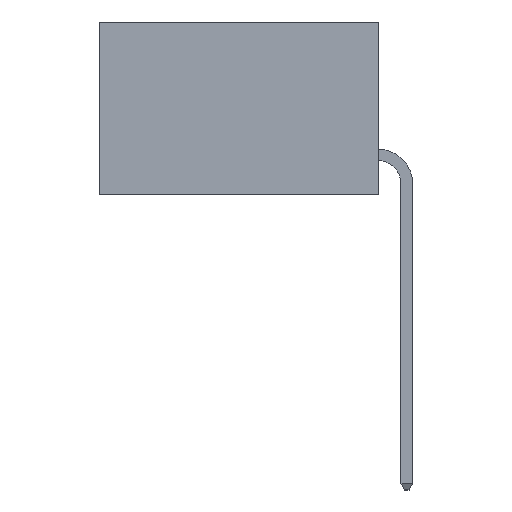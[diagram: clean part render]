
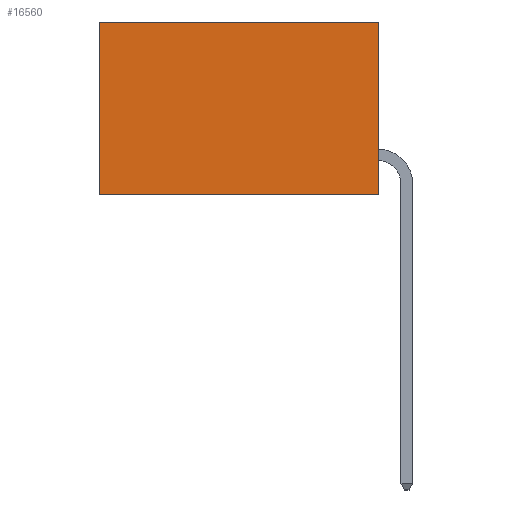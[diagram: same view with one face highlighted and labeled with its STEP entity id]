
A CAD part, left-side view. The second image highlights one B-rep face of the part: STEP entity #16560.
In plain terms, the highlighted planar face has unit normal (-1, 0, 0).
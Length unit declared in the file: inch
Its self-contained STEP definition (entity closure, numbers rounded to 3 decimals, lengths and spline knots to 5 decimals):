
#131 = EDGE_CURVE ( 'NONE', #2152, #14694, #21486, .T. ) ;
#343 = DIRECTION ( 'NONE',  ( 1., 0., 0. ) ) ;
#1003 = EDGE_CURVE ( 'NONE', #3513, #14694, #23149, .T. ) ;
#2152 = VERTEX_POINT ( 'NONE', #16942 ) ;
#2311 = VECTOR ( 'NONE', #14885, 39.37008 ) ;
#3032 = CARTESIAN_POINT ( 'NONE',  ( 0.2615, 0.6, -0.37 ) ) ;
#3037 = DIRECTION ( 'NONE',  ( 0., 0., -1. ) ) ;
#3513 = VERTEX_POINT ( 'NONE', #15687 ) ;
#5598 = EDGE_LOOP ( 'NONE', ( #9475, #20190, #12662, #16012 ) ) ;
#6235 = LINE ( 'NONE', #6883, #15037 ) ;
#6883 = CARTESIAN_POINT ( 'NONE',  ( 0.2615, 0., -0.37 ) ) ;
#7285 = CARTESIAN_POINT ( 'NONE',  ( 0.2615, 0., 0. ) ) ;
#8796 = DIRECTION ( 'NONE',  ( 0., 0., -1. ) ) ;
#9221 = DIRECTION ( 'NONE',  ( 0., 1., 0. ) ) ;
#9475 = ORIENTED_EDGE ( 'NONE', *, *, #1003, .T. ) ;
#12662 = ORIENTED_EDGE ( 'NONE', *, *, #21463, .F. ) ;
#12828 = AXIS2_PLACEMENT_3D ( 'NONE', #22611, #343, #13540 ) ;
#13540 = DIRECTION ( 'NONE',  ( 0., 0., -1. ) ) ;
#14694 = VERTEX_POINT ( 'NONE', #15408 ) ;
#14840 = CARTESIAN_POINT ( 'NONE',  ( 0.2615, 0., -0.37 ) ) ;
#14885 = DIRECTION ( 'NONE',  ( 0., 1., 0. ) ) ;
#14940 = LINE ( 'NONE', #7285, #23425 ) ;
#15037 = VECTOR ( 'NONE', #8796, 39.37008 ) ;
#15408 = CARTESIAN_POINT ( 'NONE',  ( 0.2615, 0.6, -0.37 ) ) ;
#15687 = CARTESIAN_POINT ( 'NONE',  ( 0.2615, 0.6, 0. ) ) ;
#16012 = ORIENTED_EDGE ( 'NONE', *, *, #17942, .T. ) ;
#16423 = FACE_OUTER_BOUND ( 'NONE', #5598, .T. ) ;
#16560 = ADVANCED_FACE ( 'NONE', ( #16423 ), #18972, .F. ) ;
#16942 = CARTESIAN_POINT ( 'NONE',  ( 0.2615, 0., -0.37 ) ) ;
#16950 = CARTESIAN_POINT ( 'NONE',  ( 0.2615, 0., 0. ) ) ;
#17942 = EDGE_CURVE ( 'NONE', #18062, #3513, #14940, .T. ) ;
#18062 = VERTEX_POINT ( 'NONE', #16950 ) ;
#18346 = VECTOR ( 'NONE', #3037, 39.37008 ) ;
#18972 = PLANE ( 'NONE',  #12828 ) ;
#20190 = ORIENTED_EDGE ( 'NONE', *, *, #131, .F. ) ;
#21463 = EDGE_CURVE ( 'NONE', #18062, #2152, #6235, .T. ) ;
#21486 = LINE ( 'NONE', #14840, #2311 ) ;
#22611 = CARTESIAN_POINT ( 'NONE',  ( 0.2615, 0., -0.37 ) ) ;
#23149 = LINE ( 'NONE', #3032, #18346 ) ;
#23425 = VECTOR ( 'NONE', #9221, 39.37008 ) ;
